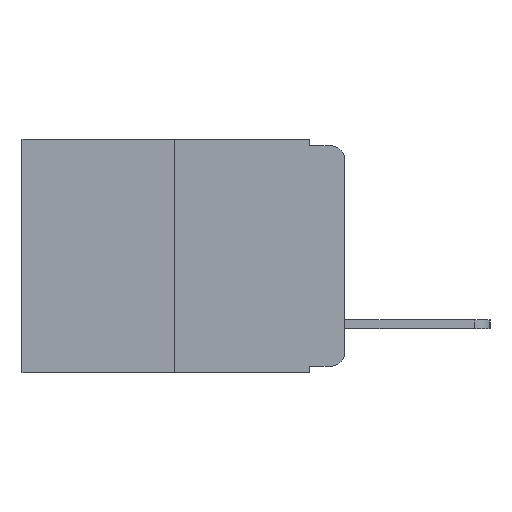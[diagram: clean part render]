
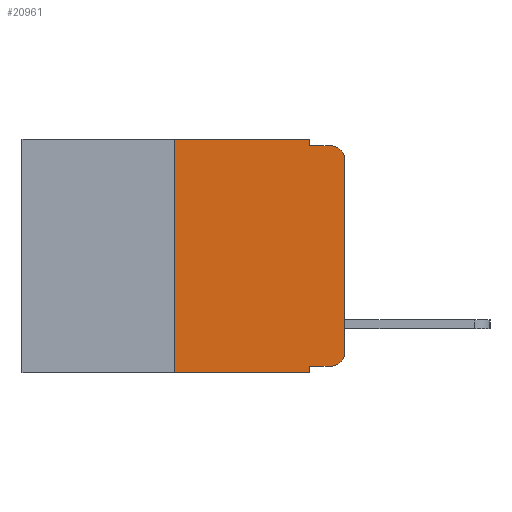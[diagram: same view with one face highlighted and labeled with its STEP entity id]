
A CAD part, left-side view. The second image highlights one B-rep face of the part: STEP entity #20961.
In plain terms, the highlighted planar face has unit normal (-1, 0, 0).
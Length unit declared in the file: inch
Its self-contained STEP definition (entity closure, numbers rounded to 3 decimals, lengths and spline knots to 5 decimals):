
#292 = EDGE_CURVE ( 'NONE', #16455, #12099, #587, .T. ) ;
#413 = CARTESIAN_POINT ( 'NONE',  ( 0., 0.02, -0.03 ) ) ;
#424 = CARTESIAN_POINT ( 'NONE',  ( 0., 0.473, 0. ) ) ;
#587 = LINE ( 'NONE', #4202, #13923 ) ;
#1268 = VECTOR ( 'NONE', #20230, 39.37008 ) ;
#1327 = LINE ( 'NONE', #8854, #4521 ) ;
#1511 = EDGE_CURVE ( 'NONE', #6108, #11817, #1671, .T. ) ;
#1671 = LINE ( 'NONE', #10440, #20300 ) ;
#2000 = PLANE ( 'NONE',  #11434 ) ;
#2247 = DIRECTION ( 'NONE',  ( 0., 0., -1. ) ) ;
#2266 = DIRECTION ( 'NONE',  ( 0., -1., 0. ) ) ;
#2556 = DIRECTION ( 'NONE',  ( 0., 0., -1. ) ) ;
#2753 = EDGE_CURVE ( 'NONE', #12395, #20511, #1327, .T. ) ;
#4015 = EDGE_CURVE ( 'NONE', #12395, #22379, #10986, .T. ) ;
#4202 = CARTESIAN_POINT ( 'NONE',  ( 0., 0.051, 0. ) ) ;
#4502 = ORIENTED_EDGE ( 'NONE', *, *, #4015, .T. ) ;
#4521 = VECTOR ( 'NONE', #2556, 39.37008 ) ;
#4690 = AXIS2_PLACEMENT_3D ( 'NONE', #18988, #14301, #14170 ) ;
#5233 = EDGE_CURVE ( 'NONE', #22379, #8079, #8157, .T. ) ;
#5529 = AXIS2_PLACEMENT_3D ( 'NONE', #413, #13098, #2247 ) ;
#6050 = DIRECTION ( 'NONE',  ( 0., 0., -1. ) ) ;
#6059 = VECTOR ( 'NONE', #9107, 39.37008 ) ;
#6086 = CARTESIAN_POINT ( 'NONE',  ( 0., 0., -0.03 ) ) ;
#6108 = VERTEX_POINT ( 'NONE', #17197 ) ;
#6517 = ORIENTED_EDGE ( 'NONE', *, *, #22429, .F. ) ;
#7085 = ORIENTED_EDGE ( 'NONE', *, *, #292, .F. ) ;
#7163 = LINE ( 'NONE', #9711, #16134 ) ;
#7568 = DIRECTION ( 'NONE',  ( 0., 0., -1. ) ) ;
#7823 = DIRECTION ( 'NONE',  ( 0., 0., 1. ) ) ;
#7903 = VERTEX_POINT ( 'NONE', #10442 ) ;
#8079 = VERTEX_POINT ( 'NONE', #14630 ) ;
#8157 = CIRCLE ( 'NONE', #4690, 0.02 ) ;
#8227 = ORIENTED_EDGE ( 'NONE', *, *, #15225, .F. ) ;
#8309 = EDGE_LOOP ( 'NONE', ( #10738, #20222, #6517, #7085, #8227, #12938, #17701, #22943, #4502, #9339 ) ) ;
#8854 = CARTESIAN_POINT ( 'NONE',  ( 0., 0.051, 0. ) ) ;
#9041 = EDGE_CURVE ( 'NONE', #6108, #20511, #20943, .T. ) ;
#9107 = DIRECTION ( 'NONE',  ( 0., -1., 0. ) ) ;
#9339 = ORIENTED_EDGE ( 'NONE', *, *, #5233, .T. ) ;
#9562 = DIRECTION ( 'NONE',  ( 0., 0., 1. ) ) ;
#9711 = CARTESIAN_POINT ( 'NONE',  ( 0., 0., 0. ) ) ;
#9987 = CARTESIAN_POINT ( 'NONE',  ( 0., 0.051, -0.333 ) ) ;
#10304 = LINE ( 'NONE', #19803, #6059 ) ;
#10440 = CARTESIAN_POINT ( 'NONE',  ( 0., 0.25, 0. ) ) ;
#10442 = CARTESIAN_POINT ( 'NONE',  ( 0., 0.02, -0.01 ) ) ;
#10654 = FACE_OUTER_BOUND ( 'NONE', #8309, .T. ) ;
#10738 = ORIENTED_EDGE ( 'NONE', *, *, #18927, .T. ) ;
#10986 = LINE ( 'NONE', #9987, #1268 ) ;
#11434 = AXIS2_PLACEMENT_3D ( 'NONE', #21734, #18263, #7568 ) ;
#11501 = CARTESIAN_POINT ( 'NONE',  ( 0., 0.051, -0.343 ) ) ;
#11817 = VERTEX_POINT ( 'NONE', #20390 ) ;
#12099 = VERTEX_POINT ( 'NONE', #22425 ) ;
#12395 = VERTEX_POINT ( 'NONE', #19834 ) ;
#12938 = ORIENTED_EDGE ( 'NONE', *, *, #1511, .F. ) ;
#13098 = DIRECTION ( 'NONE',  ( -1., 0., 0. ) ) ;
#13495 = LINE ( 'NONE', #424, #22386 ) ;
#13732 = VERTEX_POINT ( 'NONE', #6086 ) ;
#13923 = VECTOR ( 'NONE', #6050, 39.37008 ) ;
#14170 = DIRECTION ( 'NONE',  ( 0., 0., -1. ) ) ;
#14301 = DIRECTION ( 'NONE',  ( -1., 0., 0. ) ) ;
#14630 = CARTESIAN_POINT ( 'NONE',  ( 0., 0., -0.313 ) ) ;
#15225 = EDGE_CURVE ( 'NONE', #11817, #16455, #13495, .T. ) ;
#16073 = CARTESIAN_POINT ( 'NONE',  ( 0., 0.02, -0.333 ) ) ;
#16134 = VECTOR ( 'NONE', #7823, 39.37008 ) ;
#16233 = VECTOR ( 'NONE', #21200, 39.37008 ) ;
#16455 = VERTEX_POINT ( 'NONE', #20253 ) ;
#17197 = CARTESIAN_POINT ( 'NONE',  ( 0., 0.25, -0.343 ) ) ;
#17701 = ORIENTED_EDGE ( 'NONE', *, *, #9041, .T. ) ;
#18263 = DIRECTION ( 'NONE',  ( 1., 0., 0. ) ) ;
#18927 = EDGE_CURVE ( 'NONE', #8079, #13732, #7163, .T. ) ;
#18988 = CARTESIAN_POINT ( 'NONE',  ( 0., 0.02, -0.313 ) ) ;
#19418 = CIRCLE ( 'NONE', #5529, 0.02 ) ;
#19803 = CARTESIAN_POINT ( 'NONE',  ( 0., 0.051, -0.01 ) ) ;
#19834 = CARTESIAN_POINT ( 'NONE',  ( 0., 0.051, -0.333 ) ) ;
#20106 = EDGE_CURVE ( 'NONE', #13732, #7903, #19418, .T. ) ;
#20222 = ORIENTED_EDGE ( 'NONE', *, *, #20106, .T. ) ;
#20230 = DIRECTION ( 'NONE',  ( 0., -1., 0. ) ) ;
#20253 = CARTESIAN_POINT ( 'NONE',  ( 0., 0.051, 0. ) ) ;
#20300 = VECTOR ( 'NONE', #9562, 39.37008 ) ;
#20390 = CARTESIAN_POINT ( 'NONE',  ( 0., 0.25, 0. ) ) ;
#20511 = VERTEX_POINT ( 'NONE', #11501 ) ;
#20943 = LINE ( 'NONE', #21275, #16233 ) ;
#20961 = ADVANCED_FACE ( 'NONE', ( #10654 ), #2000, .F. ) ;
#21200 = DIRECTION ( 'NONE',  ( 0., -1., 0. ) ) ;
#21275 = CARTESIAN_POINT ( 'NONE',  ( 0., 0.473, -0.343 ) ) ;
#21734 = CARTESIAN_POINT ( 'NONE',  ( 0., 0.473, 0. ) ) ;
#22379 = VERTEX_POINT ( 'NONE', #16073 ) ;
#22386 = VECTOR ( 'NONE', #2266, 39.37008 ) ;
#22425 = CARTESIAN_POINT ( 'NONE',  ( 0., 0.051, -0.01 ) ) ;
#22429 = EDGE_CURVE ( 'NONE', #12099, #7903, #10304, .T. ) ;
#22943 = ORIENTED_EDGE ( 'NONE', *, *, #2753, .F. ) ;
